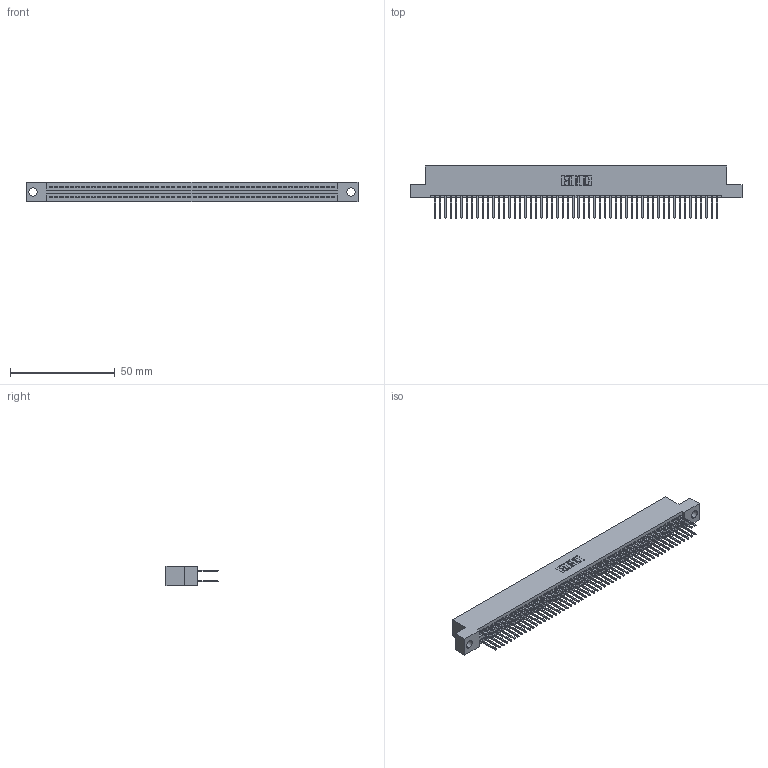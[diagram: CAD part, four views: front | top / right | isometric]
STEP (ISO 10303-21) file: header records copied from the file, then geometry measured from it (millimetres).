
FILE_DESCRIPTION (( 'STEP AP203' ), '1' );
FILE_NAME ('395-108-523-204.STEP', '2021-06-17T17:00:08', ( '' ), ( '' ), 'SwSTEP 2.0', 'SolidWorks 2020', '' );
FILE_SCHEMA (( 'CONFIG_CONTROL_DESIGN' ));
Length unit declared in the file: inch
Products named in the file (3): 345-292-001_345-293-123; 395-108-523-204; 345 Part_Flush Mounting Lugs - 0.156 Dia-TI
Assembly tree (109 placements, depth 2):
  395-108-523-204
    345 Part_Flush Mounting Lugs - 0.156 Dia-TI
    345-292-001_345-293-123  x108
Bounding box: 158.37 x 24.82 x 9.4 mm (x, y, z)
Volume: 15611 mm3; surface area: 24152.6 mm2
Topology: 109 solids, 109 shells, 5540 faces, 16469 edges, 10834 vertices
Faces by surface type: plane 3658, cylinder 1882
Entity records: 41191 total; most frequent: CARTESIAN_POINT 6898, ORIENTED_EDGE 6830, DIRECTION 6067, EDGE_CURVE 3415, VECTOR 3067, LINE 3067, VERTEX_POINT 2274, AXIS2_PLACEMENT_3D 1500
